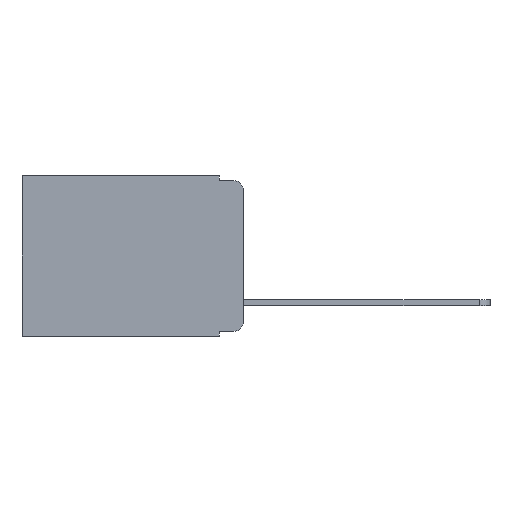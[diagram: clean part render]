
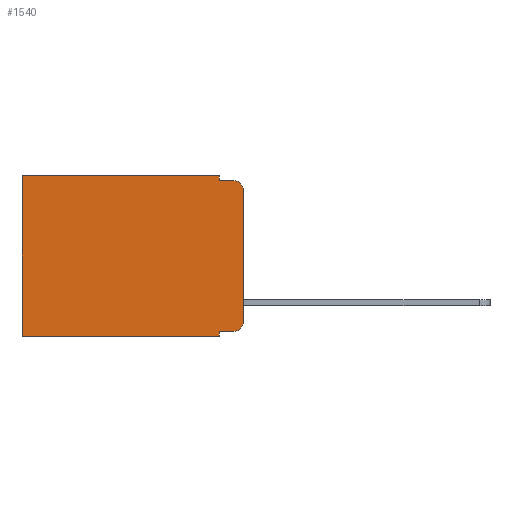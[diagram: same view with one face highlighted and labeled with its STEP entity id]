
A CAD part, left-side view. The second image highlights one B-rep face of the part: STEP entity #1540.
In plain terms, the highlighted planar face has unit normal (-1, 0, 0).
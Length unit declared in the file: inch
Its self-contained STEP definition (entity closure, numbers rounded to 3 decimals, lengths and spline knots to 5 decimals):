
#33 = ORIENTED_EDGE ( 'NONE', *, *, #7802, .T. ) ;
#134 = VERTEX_POINT ( 'NONE', #6141 ) ;
#173 = LINE ( 'NONE', #3872, #8212 ) ;
#380 = EDGE_CURVE ( 'NONE', #1105, #4343, #173, .T. ) ;
#399 = EDGE_CURVE ( 'NONE', #1105, #3372, #8911, .T. ) ;
#488 = VECTOR ( 'NONE', #4487, 39.37008 ) ;
#564 = VERTEX_POINT ( 'NONE', #3109 ) ;
#580 = DIRECTION ( 'NONE',  ( 0., 0., -1. ) ) ;
#594 = CARTESIAN_POINT ( 'NONE',  ( 0.298, 0.02, -0.313 ) ) ;
#795 = VERTEX_POINT ( 'NONE', #3305 ) ;
#972 = CARTESIAN_POINT ( 'NONE',  ( 0.298, 0., 0. ) ) ;
#1105 = VERTEX_POINT ( 'NONE', #7853 ) ;
#1211 = DIRECTION ( 'NONE',  ( -1., 0., 0. ) ) ;
#1244 = EDGE_CURVE ( 'NONE', #134, #3771, #4901, .T. ) ;
#1491 = ORIENTED_EDGE ( 'NONE', *, *, #380, .F. ) ;
#1511 = DIRECTION ( 'NONE',  ( 0., 1., 0. ) ) ;
#1540 = ADVANCED_FACE ( 'NONE', ( #8011 ), #4498, .F. ) ;
#1648 = VERTEX_POINT ( 'NONE', #1949 ) ;
#1769 = ORIENTED_EDGE ( 'NONE', *, *, #399, .T. ) ;
#1912 = EDGE_CURVE ( 'NONE', #564, #795, #5092, .T. ) ;
#1949 = CARTESIAN_POINT ( 'NONE',  ( 0.298, 0.051, -0.01 ) ) ;
#1957 = DIRECTION ( 'NONE',  ( -1., 0., 0. ) ) ;
#2004 = CARTESIAN_POINT ( 'NONE',  ( 0.298, 0.02, -0.03 ) ) ;
#2032 = ORIENTED_EDGE ( 'NONE', *, *, #1244, .T. ) ;
#2209 = LINE ( 'NONE', #2582, #5913 ) ;
#2255 = EDGE_CURVE ( 'NONE', #564, #6471, #2209, .T. ) ;
#2283 = VERTEX_POINT ( 'NONE', #7581 ) ;
#2582 = CARTESIAN_POINT ( 'NONE',  ( 0.298, 0.051, 0. ) ) ;
#2733 = DIRECTION ( 'NONE',  ( 0., 0., -1. ) ) ;
#2783 = DIRECTION ( 'NONE',  ( 1., 0., 0. ) ) ;
#2853 = CARTESIAN_POINT ( 'NONE',  ( 0.298, 0., -0.343 ) ) ;
#2882 = DIRECTION ( 'NONE',  ( 0., 0., -1. ) ) ;
#3085 = VECTOR ( 'NONE', #7387, 39.37008 ) ;
#3109 = CARTESIAN_POINT ( 'NONE',  ( 0.298, 0.051, -0.333 ) ) ;
#3305 = CARTESIAN_POINT ( 'NONE',  ( 0.298, 0.02, -0.333 ) ) ;
#3372 = VERTEX_POINT ( 'NONE', #8590 ) ;
#3771 = VERTEX_POINT ( 'NONE', #4101 ) ;
#3795 = LINE ( 'NONE', #3814, #8484 ) ;
#3814 = CARTESIAN_POINT ( 'NONE',  ( 0.298, 0.051, 0. ) ) ;
#3872 = CARTESIAN_POINT ( 'NONE',  ( 0.298, 0., 0. ) ) ;
#3878 = ORIENTED_EDGE ( 'NONE', *, *, #3986, .T. ) ;
#3986 = EDGE_CURVE ( 'NONE', #2283, #134, #5104, .T. ) ;
#4088 = EDGE_LOOP ( 'NONE', ( #1491, #1769, #5572, #8857, #3878, #2032, #4359, #9004, #6177, #33 ) ) ;
#4101 = CARTESIAN_POINT ( 'NONE',  ( 0.298, 0.473, -0.343 ) ) ;
#4343 = VERTEX_POINT ( 'NONE', #6964 ) ;
#4359 = ORIENTED_EDGE ( 'NONE', *, *, #6187, .F. ) ;
#4452 = CARTESIAN_POINT ( 'NONE',  ( 0.298, 0.473, 0. ) ) ;
#4477 = AXIS2_PLACEMENT_3D ( 'NONE', #594, #1211, #580 ) ;
#4487 = DIRECTION ( 'NONE',  ( 0., 0., -1. ) ) ;
#4498 = PLANE ( 'NONE',  #6528 ) ;
#4786 = VECTOR ( 'NONE', #1511, 39.37008 ) ;
#4901 = LINE ( 'NONE', #4452, #488 ) ;
#5092 = LINE ( 'NONE', #6882, #8189 ) ;
#5104 = LINE ( 'NONE', #7378, #3085 ) ;
#5572 = ORIENTED_EDGE ( 'NONE', *, *, #8091, .F. ) ;
#5574 = DIRECTION ( 'NONE',  ( 0., -1., 0. ) ) ;
#5913 = VECTOR ( 'NONE', #2882, 39.37008 ) ;
#6141 = CARTESIAN_POINT ( 'NONE',  ( 0.298, 0.473, 0. ) ) ;
#6177 = ORIENTED_EDGE ( 'NONE', *, *, #1912, .T. ) ;
#6187 = EDGE_CURVE ( 'NONE', #6471, #3771, #6527, .T. ) ;
#6311 = VECTOR ( 'NONE', #7799, 39.37008 ) ;
#6471 = VERTEX_POINT ( 'NONE', #7405 ) ;
#6497 = LINE ( 'NONE', #8848, #6311 ) ;
#6527 = LINE ( 'NONE', #2853, #4786 ) ;
#6528 = AXIS2_PLACEMENT_3D ( 'NONE', #972, #2783, #2733 ) ;
#6882 = CARTESIAN_POINT ( 'NONE',  ( 0.298, 0.051, -0.333 ) ) ;
#6964 = CARTESIAN_POINT ( 'NONE',  ( 0.298, 0., -0.313 ) ) ;
#7378 = CARTESIAN_POINT ( 'NONE',  ( 0.298, 0., 0. ) ) ;
#7387 = DIRECTION ( 'NONE',  ( 0., 1., 0. ) ) ;
#7405 = CARTESIAN_POINT ( 'NONE',  ( 0.298, 0.051, -0.343 ) ) ;
#7437 = CIRCLE ( 'NONE', #4477, 0.02 ) ;
#7453 = AXIS2_PLACEMENT_3D ( 'NONE', #2004, #1957, #7861 ) ;
#7581 = CARTESIAN_POINT ( 'NONE',  ( 0.298, 0.051, 0. ) ) ;
#7799 = DIRECTION ( 'NONE',  ( 0., -1., 0. ) ) ;
#7802 = EDGE_CURVE ( 'NONE', #795, #4343, #7437, .T. ) ;
#7853 = CARTESIAN_POINT ( 'NONE',  ( 0.298, 0., -0.03 ) ) ;
#7861 = DIRECTION ( 'NONE',  ( 0., 0., -1. ) ) ;
#7944 = EDGE_CURVE ( 'NONE', #2283, #1648, #3795, .T. ) ;
#8011 = FACE_OUTER_BOUND ( 'NONE', #4088, .T. ) ;
#8091 = EDGE_CURVE ( 'NONE', #1648, #3372, #6497, .T. ) ;
#8127 = DIRECTION ( 'NONE',  ( 0., 0., -1. ) ) ;
#8189 = VECTOR ( 'NONE', #5574, 39.37008 ) ;
#8212 = VECTOR ( 'NONE', #8921, 39.37008 ) ;
#8484 = VECTOR ( 'NONE', #8127, 39.37008 ) ;
#8590 = CARTESIAN_POINT ( 'NONE',  ( 0.298, 0.02, -0.01 ) ) ;
#8848 = CARTESIAN_POINT ( 'NONE',  ( 0.298, 0.051, -0.01 ) ) ;
#8857 = ORIENTED_EDGE ( 'NONE', *, *, #7944, .F. ) ;
#8911 = CIRCLE ( 'NONE', #7453, 0.02 ) ;
#8921 = DIRECTION ( 'NONE',  ( 0., 0., -1. ) ) ;
#9004 = ORIENTED_EDGE ( 'NONE', *, *, #2255, .F. ) ;
